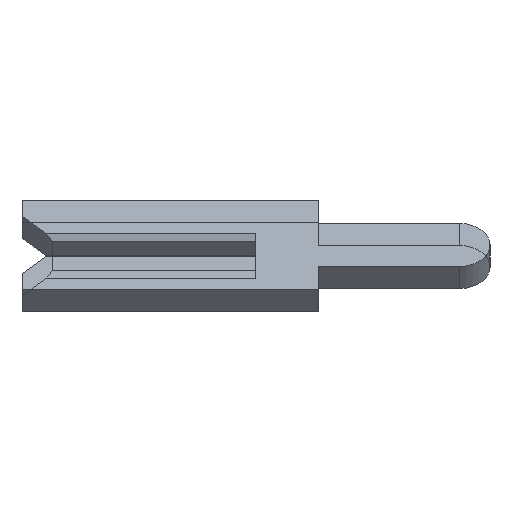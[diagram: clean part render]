
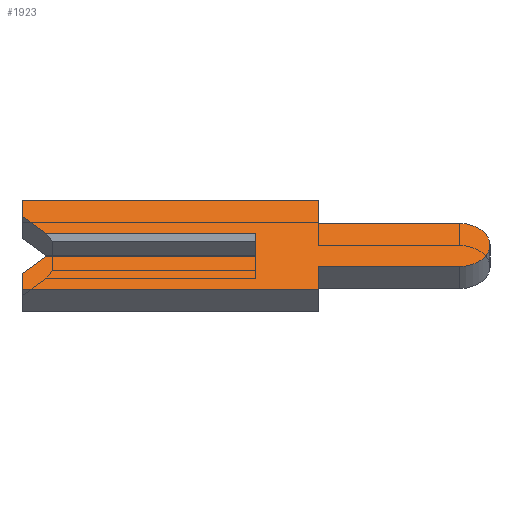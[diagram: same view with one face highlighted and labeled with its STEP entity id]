
A CAD part, left-side view. The second image highlights one B-rep face of the part: STEP entity #1923.
In plain terms, the highlighted face is planar.
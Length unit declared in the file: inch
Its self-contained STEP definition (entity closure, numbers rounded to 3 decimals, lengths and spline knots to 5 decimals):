
#60 = LINE ( 'NONE', #2564, #225 ) ;
#71 = CARTESIAN_POINT ( 'NONE',  ( -0.01, 0.134, 0.01 ) ) ;
#157 = VERTEX_POINT ( 'NONE', #4191 ) ;
#181 = ORIENTED_EDGE ( 'NONE', *, *, #2818, .F. ) ;
#203 = VERTEX_POINT ( 'NONE', #3549 ) ;
#222 = LINE ( 'NONE', #3410, #2556 ) ;
#225 = VECTOR ( 'NONE', #3964, 39.37008 ) ;
#257 = EDGE_CURVE ( 'NONE', #157, #4051, #1897, .T. ) ;
#288 = VECTOR ( 'NONE', #3880, 39.37008 ) ;
#334 = VERTEX_POINT ( 'NONE', #3531 ) ;
#347 = EDGE_CURVE ( 'NONE', #2896, #4032, #3982, .T. ) ;
#359 = ORIENTED_EDGE ( 'NONE', *, *, #1218, .F. ) ;
#415 = ORIENTED_EDGE ( 'NONE', *, *, #4012, .F. ) ;
#439 = VECTOR ( 'NONE', #2195, 39.37008 ) ;
#457 = CARTESIAN_POINT ( 'NONE',  ( -0.01, -0.04, -0.04 ) ) ;
#531 = DIRECTION ( 'NONE',  ( 0., -1., 0. ) ) ;
#609 = ORIENTED_EDGE ( 'NONE', *, *, #1125, .F. ) ;
#618 = CARTESIAN_POINT ( 'NONE',  ( -0.01, 0., -0.01 ) ) ;
#629 = CARTESIAN_POINT ( 'NONE',  ( -0.01, -0.04, 0.0195 ) ) ;
#646 = EDGE_CURVE ( 'NONE', #2750, #4188, #2290, .T. ) ;
#659 = ORIENTED_EDGE ( 'NONE', *, *, #2584, .F. ) ;
#663 = CARTESIAN_POINT ( 'NONE',  ( -0.01, 0.15, -0.026 ) ) ;
#701 = DIRECTION ( 'NONE',  ( 0., -1., 0. ) ) ;
#765 = DIRECTION ( 'NONE',  ( 0., 1., 0. ) ) ;
#776 = ORIENTED_EDGE ( 'NONE', *, *, #3295, .F. ) ;
#825 = CARTESIAN_POINT ( 'NONE',  ( -0.01, 0.15, 0.026 ) ) ;
#869 = CARTESIAN_POINT ( 'NONE',  ( -0.01, 0.15, 0.01 ) ) ;
#900 = DIRECTION ( 'NONE',  ( 0., 0., -1. ) ) ;
#956 = CARTESIAN_POINT ( 'NONE',  ( -0.01, -0.1305, 0. ) ) ;
#1062 = CARTESIAN_POINT ( 'NONE',  ( -0.01, -0.04, -0.0195 ) ) ;
#1125 = EDGE_CURVE ( 'NONE', #4188, #2506, #3055, .T. ) ;
#1187 = CARTESIAN_POINT ( 'NONE',  ( -0.01, 0.15, -0.04 ) ) ;
#1210 = VECTOR ( 'NONE', #3005, 39.37008 ) ;
#1218 = EDGE_CURVE ( 'NONE', #2506, #157, #2067, .T. ) ;
#1219 = LINE ( 'NONE', #1971, #1270 ) ;
#1252 = ORIENTED_EDGE ( 'NONE', *, *, #1353, .F. ) ;
#1268 = VERTEX_POINT ( 'NONE', #825 ) ;
#1270 = VECTOR ( 'NONE', #1313, 39.37008 ) ;
#1278 = VERTEX_POINT ( 'NONE', #71 ) ;
#1299 = ORIENTED_EDGE ( 'NONE', *, *, #3174, .F. ) ;
#1313 = DIRECTION ( 'NONE',  ( 0., -1., 0. ) ) ;
#1353 = EDGE_CURVE ( 'NONE', #3493, #203, #60, .T. ) ;
#1370 = CARTESIAN_POINT ( 'NONE',  ( -0.01, -0.04, -0.0195 ) ) ;
#1377 = VECTOR ( 'NONE', #1488, 39.37008 ) ;
#1401 = DIRECTION ( 'NONE',  ( 0., -1., 0. ) ) ;
#1425 = DIRECTION ( 'NONE',  ( 0., 0., 1. ) ) ;
#1488 = DIRECTION ( 'NONE',  ( 0., 1., 0. ) ) ;
#1621 = CARTESIAN_POINT ( 'NONE',  ( -0.01, -0.04, 0.04 ) ) ;
#1636 = CARTESIAN_POINT ( 'NONE',  ( -0.01, 0.15, 0.026 ) ) ;
#1663 = DIRECTION ( 'NONE',  ( 0., 0., -1. ) ) ;
#1746 = EDGE_CURVE ( 'NONE', #1278, #203, #3577, .T. ) ;
#1839 = EDGE_CURVE ( 'NONE', #4051, #334, #3636, .T. ) ;
#1897 = LINE ( 'NONE', #3513, #3259 ) ;
#1923 = ADVANCED_FACE ( 'NONE', ( #3962 ), #3672, .F. ) ;
#1971 = CARTESIAN_POINT ( 'NONE',  ( -0.01, -0.1305, -0.01 ) ) ;
#2030 = CARTESIAN_POINT ( 'NONE',  ( -0.01, 0.15, 0.04 ) ) ;
#2067 = LINE ( 'NONE', #1187, #1377 ) ;
#2100 = CARTESIAN_POINT ( 'NONE',  ( -0.01, 0.1305, 0.0065 ) ) ;
#2102 = ORIENTED_EDGE ( 'NONE', *, *, #1746, .T. ) ;
#2195 = DIRECTION ( 'NONE',  ( 0., 0., -1. ) ) ;
#2281 = VERTEX_POINT ( 'NONE', #1621 ) ;
#2283 = DIRECTION ( 'NONE',  ( 0., -0.707, 0.707 ) ) ;
#2290 = LINE ( 'NONE', #1062, #2780 ) ;
#2478 = LINE ( 'NONE', #2030, #3797 ) ;
#2506 = VERTEX_POINT ( 'NONE', #4392 ) ;
#2556 = VECTOR ( 'NONE', #1663, 39.37008 ) ;
#2564 = CARTESIAN_POINT ( 'NONE',  ( -0.01, 0., 0.0065 ) ) ;
#2584 = EDGE_CURVE ( 'NONE', #1268, #4401, #3477, .T. ) ;
#2662 = DIRECTION ( 'NONE',  ( 1., 0., 0. ) ) ;
#2750 = VERTEX_POINT ( 'NONE', #3382 ) ;
#2773 = VECTOR ( 'NONE', #701, 39.37008 ) ;
#2780 = VECTOR ( 'NONE', #765, 39.37008 ) ;
#2781 = ORIENTED_EDGE ( 'NONE', *, *, #646, .F. ) ;
#2818 = EDGE_CURVE ( 'NONE', #4032, #2750, #3927, .T. ) ;
#2896 = VERTEX_POINT ( 'NONE', #629 ) ;
#2904 = ORIENTED_EDGE ( 'NONE', *, *, #1839, .F. ) ;
#3005 = DIRECTION ( 'NONE',  ( 0., 0., 1. ) ) ;
#3055 = LINE ( 'NONE', #457, #439 ) ;
#3066 = LINE ( 'NONE', #2100, #288 ) ;
#3158 = CARTESIAN_POINT ( 'NONE',  ( -0.01, 0.15, 0.04 ) ) ;
#3174 = EDGE_CURVE ( 'NONE', #334, #3493, #1219, .T. ) ;
#3259 = VECTOR ( 'NONE', #1425, 39.37008 ) ;
#3295 = EDGE_CURVE ( 'NONE', #2281, #2896, #222, .T. ) ;
#3324 = ORIENTED_EDGE ( 'NONE', *, *, #257, .F. ) ;
#3332 = CARTESIAN_POINT ( 'NONE',  ( -0.01, 0.1305, -0.0065 ) ) ;
#3361 = DIRECTION ( 'NONE',  ( 0., 0., -1. ) ) ;
#3382 = CARTESIAN_POINT ( 'NONE',  ( -0.01, -0.1305, -0.0195 ) ) ;
#3410 = CARTESIAN_POINT ( 'NONE',  ( -0.01, -0.04, 0.04 ) ) ;
#3477 = LINE ( 'NONE', #1636, #1210 ) ;
#3478 = AXIS2_PLACEMENT_3D ( 'NONE', #956, #2662, #3361 ) ;
#3493 = VERTEX_POINT ( 'NONE', #618 ) ;
#3501 = AXIS2_PLACEMENT_3D ( 'NONE', #4057, #4015, #900 ) ;
#3513 = CARTESIAN_POINT ( 'NONE',  ( -0.01, 0.15, -0.026 ) ) ;
#3514 = VECTOR ( 'NONE', #2283, 39.37008 ) ;
#3531 = CARTESIAN_POINT ( 'NONE',  ( -0.01, 0.134, -0.01 ) ) ;
#3549 = CARTESIAN_POINT ( 'NONE',  ( -0.01, 0., 0.01 ) ) ;
#3556 = EDGE_LOOP ( 'NONE', ( #2102, #1252, #1299, #2904, #3324, #359, #609, #2781, #181, #4107, #776, #415, #659, #3776 ) ) ;
#3577 = LINE ( 'NONE', #869, #4388 ) ;
#3636 = LINE ( 'NONE', #3332, #3514 ) ;
#3672 = PLANE ( 'NONE',  #3501 ) ;
#3776 = ORIENTED_EDGE ( 'NONE', *, *, #4318, .F. ) ;
#3797 = VECTOR ( 'NONE', #1401, 39.37008 ) ;
#3866 = CARTESIAN_POINT ( 'NONE',  ( -0.01, -0.04, 0.0195 ) ) ;
#3880 = DIRECTION ( 'NONE',  ( 0., 0.707, 0.707 ) ) ;
#3927 = CIRCLE ( 'NONE', #3478, 0.0195 ) ;
#3962 = FACE_OUTER_BOUND ( 'NONE', #3556, .T. ) ;
#3964 = DIRECTION ( 'NONE',  ( 0., 0., 1. ) ) ;
#3982 = LINE ( 'NONE', #3866, #2773 ) ;
#4012 = EDGE_CURVE ( 'NONE', #4401, #2281, #2478, .T. ) ;
#4015 = DIRECTION ( 'NONE',  ( 1., 0., 0. ) ) ;
#4032 = VERTEX_POINT ( 'NONE', #4127 ) ;
#4051 = VERTEX_POINT ( 'NONE', #663 ) ;
#4057 = CARTESIAN_POINT ( 'NONE',  ( -0.01, -0.1305, 0. ) ) ;
#4107 = ORIENTED_EDGE ( 'NONE', *, *, #347, .F. ) ;
#4127 = CARTESIAN_POINT ( 'NONE',  ( -0.01, -0.1305, 0.0195 ) ) ;
#4188 = VERTEX_POINT ( 'NONE', #1370 ) ;
#4191 = CARTESIAN_POINT ( 'NONE',  ( -0.01, 0.15, -0.04 ) ) ;
#4318 = EDGE_CURVE ( 'NONE', #1278, #1268, #3066, .T. ) ;
#4388 = VECTOR ( 'NONE', #531, 39.37008 ) ;
#4392 = CARTESIAN_POINT ( 'NONE',  ( -0.01, -0.04, -0.04 ) ) ;
#4401 = VERTEX_POINT ( 'NONE', #3158 ) ;
